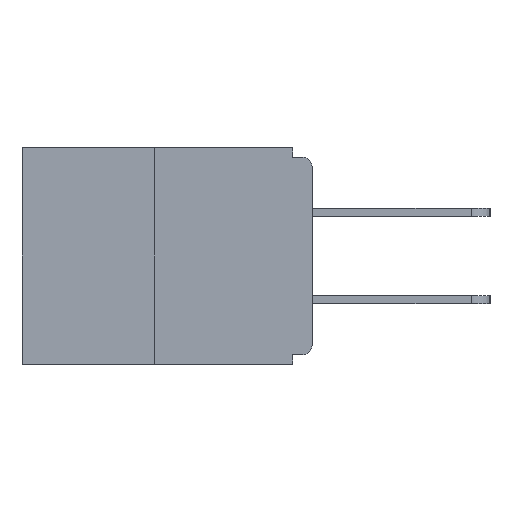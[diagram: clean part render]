
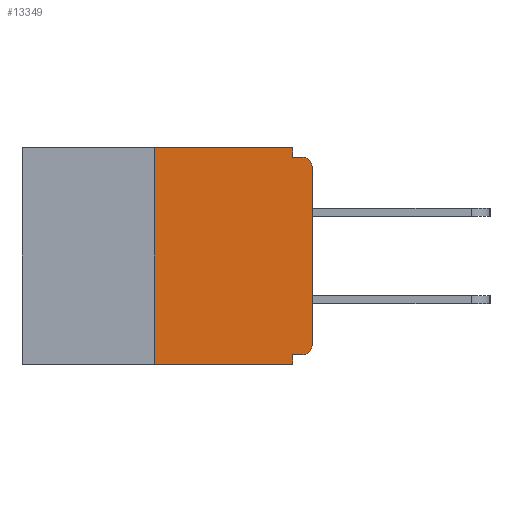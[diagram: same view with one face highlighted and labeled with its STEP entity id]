
A CAD part, left-side view. The second image highlights one B-rep face of the part: STEP entity #13349.
In plain terms, the highlighted planar face has unit normal (-1, 0, 0).
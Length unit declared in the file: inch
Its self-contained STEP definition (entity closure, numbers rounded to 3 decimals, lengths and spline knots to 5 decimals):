
#6 = LINE ( 'NONE', #18142, #18195 ) ;
#784 = CARTESIAN_POINT ( 'NONE',  ( 0., 0., -0.015 ) ) ;
#1004 = PLANE ( 'NONE',  #1863 ) ;
#1460 = VERTEX_POINT ( 'NONE', #10995 ) ;
#1476 = CARTESIAN_POINT ( 'NONE',  ( 0., 0.015, -0.03 ) ) ;
#1495 = LINE ( 'NONE', #15328, #8273 ) ;
#1607 = LINE ( 'NONE', #15175, #12196 ) ;
#1619 = VERTEX_POINT ( 'NONE', #2658 ) ;
#1659 = DIRECTION ( 'NONE',  ( -1., 0., 0. ) ) ;
#1678 = CARTESIAN_POINT ( 'NONE',  ( 0., 0.031, -0.328 ) ) ;
#1802 = EDGE_CURVE ( 'NONE', #16767, #11784, #14522, .T. ) ;
#1863 = AXIS2_PLACEMENT_3D ( 'NONE', #13823, #9521, #16762 ) ;
#2204 = CARTESIAN_POINT ( 'NONE',  ( 0., 0.46, -0.343 ) ) ;
#2214 = ORIENTED_EDGE ( 'NONE', *, *, #1802, .F. ) ;
#2302 = VERTEX_POINT ( 'NONE', #6034 ) ;
#2658 = CARTESIAN_POINT ( 'NONE',  ( 0., 0.015, -0.015 ) ) ;
#2841 = DIRECTION ( 'NONE',  ( 0., 0., -1. ) ) ;
#3064 = CARTESIAN_POINT ( 'NONE',  ( 0., 0.031, -0.343 ) ) ;
#3588 = VERTEX_POINT ( 'NONE', #11859 ) ;
#3602 = DIRECTION ( 'NONE',  ( 0., -1., 0. ) ) ;
#3655 = CARTESIAN_POINT ( 'NONE',  ( 0., 0.015, -0.313 ) ) ;
#3812 = VECTOR ( 'NONE', #10899, 39.37008 ) ;
#3959 = CARTESIAN_POINT ( 'NONE',  ( 0., 0.25, 0. ) ) ;
#3977 = EDGE_CURVE ( 'NONE', #11784, #17667, #11789, .T. ) ;
#4371 = ORIENTED_EDGE ( 'NONE', *, *, #14477, .F. ) ;
#4982 = CARTESIAN_POINT ( 'NONE',  ( 0., 0.25, 0. ) ) ;
#5096 = VECTOR ( 'NONE', #17049, 39.37008 ) ;
#5429 = EDGE_CURVE ( 'NONE', #16767, #3588, #7033, .T. ) ;
#5658 = ORIENTED_EDGE ( 'NONE', *, *, #9262, .T. ) ;
#5887 = DIRECTION ( 'NONE',  ( 0., 0., -1. ) ) ;
#6034 = CARTESIAN_POINT ( 'NONE',  ( 0., 0.25, -0.343 ) ) ;
#6295 = LINE ( 'NONE', #784, #3812 ) ;
#6922 = EDGE_CURVE ( 'NONE', #1460, #1619, #6295, .T. ) ;
#7033 = CIRCLE ( 'NONE', #17104, 0.015 ) ;
#7299 = EDGE_LOOP ( 'NONE', ( #16607, #4371, #9950, #13950, #2214, #17466, #5658, #17083, #10810, #15846 ) ) ;
#8001 = VECTOR ( 'NONE', #2841, 39.37008 ) ;
#8022 = VECTOR ( 'NONE', #3602, 39.37008 ) ;
#8273 = VECTOR ( 'NONE', #10991, 39.37008 ) ;
#8432 = FACE_OUTER_BOUND ( 'NONE', #7299, .T. ) ;
#8481 = EDGE_CURVE ( 'NONE', #15279, #1619, #15550, .T. ) ;
#8503 = VERTEX_POINT ( 'NONE', #10104 ) ;
#9262 = EDGE_CURVE ( 'NONE', #3588, #15279, #6, .T. ) ;
#9521 = DIRECTION ( 'NONE',  ( 1., 0., 0. ) ) ;
#9761 = DIRECTION ( 'NONE',  ( 0., 0., 1. ) ) ;
#9950 = ORIENTED_EDGE ( 'NONE', *, *, #12775, .T. ) ;
#10104 = CARTESIAN_POINT ( 'NONE',  ( 0., 0.031, 0. ) ) ;
#10648 = VERTEX_POINT ( 'NONE', #3959 ) ;
#10653 = VECTOR ( 'NONE', #15029, 39.37008 ) ;
#10810 = ORIENTED_EDGE ( 'NONE', *, *, #6922, .F. ) ;
#10899 = DIRECTION ( 'NONE',  ( 0., -1., 0. ) ) ;
#10991 = DIRECTION ( 'NONE',  ( 0., 0., -1. ) ) ;
#10995 = CARTESIAN_POINT ( 'NONE',  ( 0., 0.031, -0.015 ) ) ;
#11784 = VERTEX_POINT ( 'NONE', #1678 ) ;
#11789 = LINE ( 'NONE', #15736, #8001 ) ;
#11811 = LINE ( 'NONE', #4982, #10653 ) ;
#11859 = CARTESIAN_POINT ( 'NONE',  ( 0., 0., -0.313 ) ) ;
#11977 = EDGE_CURVE ( 'NONE', #8503, #1460, #1495, .T. ) ;
#12023 = AXIS2_PLACEMENT_3D ( 'NONE', #1476, #1659, #5887 ) ;
#12196 = VECTOR ( 'NONE', #12348, 39.37008 ) ;
#12348 = DIRECTION ( 'NONE',  ( 0., -1., 0. ) ) ;
#12775 = EDGE_CURVE ( 'NONE', #2302, #17667, #12937, .T. ) ;
#12937 = LINE ( 'NONE', #2204, #8022 ) ;
#12948 = CARTESIAN_POINT ( 'NONE',  ( 0., 0., -0.03 ) ) ;
#13150 = CARTESIAN_POINT ( 'NONE',  ( 0., 0.015, -0.328 ) ) ;
#13349 = ADVANCED_FACE ( 'NONE', ( #8432 ), #1004, .F. ) ;
#13711 = DIRECTION ( 'NONE',  ( 0., 0., -1. ) ) ;
#13823 = CARTESIAN_POINT ( 'NONE',  ( 0., 0.46, 0. ) ) ;
#13950 = ORIENTED_EDGE ( 'NONE', *, *, #3977, .F. ) ;
#14477 = EDGE_CURVE ( 'NONE', #2302, #10648, #11811, .T. ) ;
#14522 = LINE ( 'NONE', #15619, #5096 ) ;
#15029 = DIRECTION ( 'NONE',  ( 0., 0., 1. ) ) ;
#15175 = CARTESIAN_POINT ( 'NONE',  ( 0., 0.46, 0. ) ) ;
#15279 = VERTEX_POINT ( 'NONE', #12948 ) ;
#15328 = CARTESIAN_POINT ( 'NONE',  ( 0., 0.031, 0. ) ) ;
#15550 = CIRCLE ( 'NONE', #12023, 0.015 ) ;
#15619 = CARTESIAN_POINT ( 'NONE',  ( 0., 0., -0.328 ) ) ;
#15736 = CARTESIAN_POINT ( 'NONE',  ( 0., 0.031, -0.343 ) ) ;
#15846 = ORIENTED_EDGE ( 'NONE', *, *, #11977, .F. ) ;
#16455 = DIRECTION ( 'NONE',  ( -1., 0., 0. ) ) ;
#16607 = ORIENTED_EDGE ( 'NONE', *, *, #17502, .F. ) ;
#16762 = DIRECTION ( 'NONE',  ( 0., 0., -1. ) ) ;
#16767 = VERTEX_POINT ( 'NONE', #13150 ) ;
#17049 = DIRECTION ( 'NONE',  ( 0., 1., 0. ) ) ;
#17083 = ORIENTED_EDGE ( 'NONE', *, *, #8481, .T. ) ;
#17104 = AXIS2_PLACEMENT_3D ( 'NONE', #3655, #16455, #13711 ) ;
#17466 = ORIENTED_EDGE ( 'NONE', *, *, #5429, .T. ) ;
#17502 = EDGE_CURVE ( 'NONE', #10648, #8503, #1607, .T. ) ;
#17667 = VERTEX_POINT ( 'NONE', #3064 ) ;
#18142 = CARTESIAN_POINT ( 'NONE',  ( 0., 0., 0. ) ) ;
#18195 = VECTOR ( 'NONE', #9761, 39.37008 ) ;
